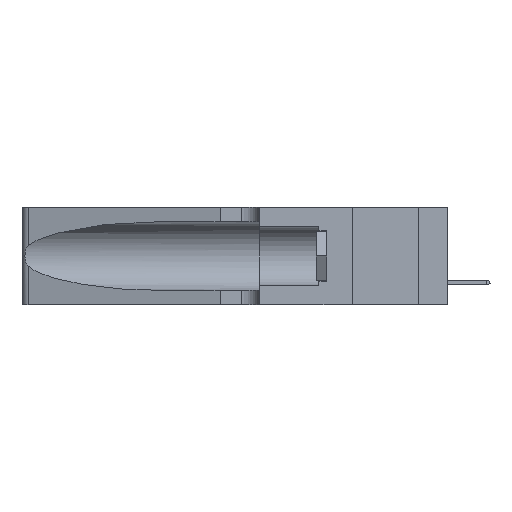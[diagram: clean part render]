
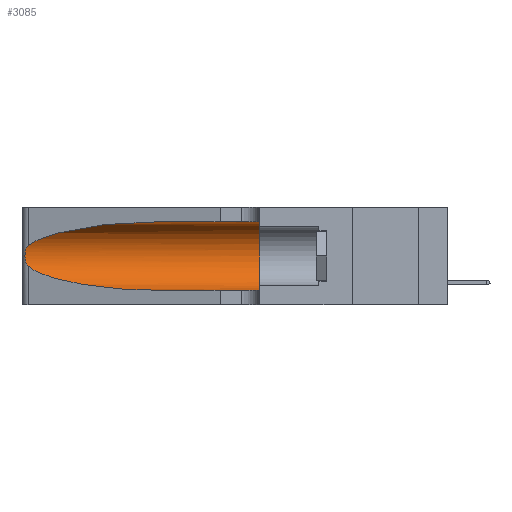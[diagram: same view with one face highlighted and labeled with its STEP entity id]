
A CAD part, left-side view. The second image highlights one B-rep face of the part: STEP entity #3085.
In plain terms, the highlighted cylindrical face has radius 3.308 mm (diameter 6.617 mm), a partial arc.
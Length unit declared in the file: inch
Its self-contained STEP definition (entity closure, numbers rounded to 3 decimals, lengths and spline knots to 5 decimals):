
#16 = CARTESIAN_POINT ( 'NONE',  ( 0.1305, 0.72297, 0.31525 ) ) ;
#90 = CARTESIAN_POINT ( 'NONE',  ( 0.25555, 1.22994, 0.2215 ) ) ;
#122 = CARTESIAN_POINT ( 'NONE',  ( 0.26018, 1.23835, 0.19895 ) ) ;
#381 = CARTESIAN_POINT ( 'NONE',  ( 0.1305, 0.72297, 0.05475 ) ) ;
#1040 = AXIS2_PLACEMENT_3D ( 'NONE', #11306, #14944, #5974 ) ;
#3085 = ADVANCED_FACE ( 'NONE', ( #10903 ), #20710, .F. ) ;
#3387 = EDGE_CURVE ( 'NONE', #22578, #42365, #36849, .T. ) ;
#4624 = DIRECTION ( 'NONE',  ( 0., -1., 0. ) ) ;
#4936 = CARTESIAN_POINT ( 'NONE',  ( 0.25789, 1.23486, 0.15765 ) ) ;
#5235 = CARTESIAN_POINT ( 'NONE',  ( 0.26075, 1.23896, 0.178 ) ) ;
#5974 = DIRECTION ( 'NONE',  ( 0., 0., -1. ) ) ;
#6119 = CARTESIAN_POINT ( 'NONE',  ( 0.25639, 1.23184, 0.21858 ) ) ;
#6278 =( BOUNDED_CURVE ( )  B_SPLINE_CURVE ( 3, ( #33936, #40013, #6441, #381 ),
 .UNSPECIFIED., .F., .F. ) 
 B_SPLINE_CURVE_WITH_KNOTS ( ( 4, 4 ),
 ( 3.44316, 4.71239 ),
 .UNSPECIFIED. ) 
 CURVE ( )  GEOMETRIC_REPRESENTATION_ITEM ( )  RATIONAL_B_SPLINE_CURVE ( ( 1., 0.87, 0.87, 1. ) ) 
 REPRESENTATION_ITEM ( '' )  );
#6441 = CARTESIAN_POINT ( 'NONE',  ( 0.18966, 0.96281, 0.05475 ) ) ;
#6988 = CARTESIAN_POINT ( 'NONE',  ( 0.18966, 0.96281, 0.31525 ) ) ;
#7153 = CARTESIAN_POINT ( 'NONE',  ( 0.2373, 1.15595, 0.28018 ) ) ;
#7646 = VERTEX_POINT ( 'NONE', #41766 ) ;
#7783 = DIRECTION ( 'NONE',  ( 0., 0., 1. ) ) ;
#8116 = CARTESIAN_POINT ( 'NONE',  ( 0.25487, 1.22718, 0.22369 ) ) ;
#9734 = EDGE_LOOP ( 'NONE', ( #28332, #10501, #30326, #34204, #14039, #30371 ) ) ;
#10501 = ORIENTED_EDGE ( 'NONE', *, *, #3387, .T. ) ;
#10881 = CARTESIAN_POINT ( 'NONE',  ( 0.1305, 0.35, 0.31525 ) ) ;
#10903 = FACE_OUTER_BOUND ( 'NONE', #9734, .T. ) ;
#10955 = CARTESIAN_POINT ( 'NONE',  ( 0.1305, 1.61858, 0.31525 ) ) ;
#11306 = CARTESIAN_POINT ( 'NONE',  ( 0.1305, 1.61858, 0.185 ) ) ;
#12125 = CIRCLE ( 'NONE', #32154, 0.13025 ) ;
#12534 = CARTESIAN_POINT ( 'NONE',  ( 0.25854, 1.2359, 0.20912 ) ) ;
#14039 = ORIENTED_EDGE ( 'NONE', *, *, #19310, .F. ) ;
#14944 = DIRECTION ( 'NONE',  ( 0., -1., 0. ) ) ;
#15349 = LINE ( 'NONE', #29283, #32809 ) ;
#15632 = CARTESIAN_POINT ( 'NONE',  ( 0.25555, 1.22993, 0.14849 ) ) ;
#17340 = CARTESIAN_POINT ( 'NONE',  ( 0.1305, 0.35, 0.185 ) ) ;
#18499 = CARTESIAN_POINT ( 'NONE',  ( 0.1305, 0.72297, 0.31525 ) ) ;
#18615 = VERTEX_POINT ( 'NONE', #10881 ) ;
#19087 = CARTESIAN_POINT ( 'NONE',  ( 0.25787, 1.23484, 0.2124 ) ) ;
#19310 = EDGE_CURVE ( 'NONE', #18615, #7646, #12125, .T. ) ;
#19911 = DIRECTION ( 'NONE',  ( 0., -1., 0. ) ) ;
#20242 = CARTESIAN_POINT ( 'NONE',  ( 0.25487, 1.22718, 0.14631 ) ) ;
#20567 = CARTESIAN_POINT ( 'NONE',  ( 0.26075, 1.23896, 0.19203 ) ) ;
#20623 = EDGE_CURVE ( 'NONE', #40345, #18615, #25537, .T. ) ;
#20710 = CYLINDRICAL_SURFACE ( 'NONE', #1040, 0.13025 ) ;
#21371 = VERTEX_POINT ( 'NONE', #37599 ) ;
#22578 = VERTEX_POINT ( 'NONE', #8116 ) ;
#23713 = EDGE_CURVE ( 'NONE', #42365, #21371, #6278, .T. ) ;
#24273 =( BOUNDED_CURVE ( )  B_SPLINE_CURVE ( 3, ( #16, #6988, #7153, #33063 ),
 .UNSPECIFIED., .F., .F. ) 
 B_SPLINE_CURVE_WITH_KNOTS ( ( 4, 4 ),
 ( 1.5708, 2.84003 ),
 .UNSPECIFIED. ) 
 CURVE ( )  GEOMETRIC_REPRESENTATION_ITEM ( )  RATIONAL_B_SPLINE_CURVE ( ( 1., 0.87, 0.87, 1. ) ) 
 REPRESENTATION_ITEM ( '' )  );
#25320 = CARTESIAN_POINT ( 'NONE',  ( 0.26017, 1.23833, 0.17102 ) ) ;
#25446 = CARTESIAN_POINT ( 'NONE',  ( 0.25487, 1.22718, 0.14631 ) ) ;
#25537 = LINE ( 'NONE', #10955, #41944 ) ;
#28332 = ORIENTED_EDGE ( 'NONE', *, *, #40671, .T. ) ;
#29283 = CARTESIAN_POINT ( 'NONE',  ( 0.1305, 1.61858, 0.05475 ) ) ;
#30326 = ORIENTED_EDGE ( 'NONE', *, *, #23713, .T. ) ;
#30371 = ORIENTED_EDGE ( 'NONE', *, *, #20623, .F. ) ;
#31306 = CARTESIAN_POINT ( 'NONE',  ( 0.25639, 1.23186, 0.15144 ) ) ;
#32154 = AXIS2_PLACEMENT_3D ( 'NONE', #17340, #40458, #7783 ) ;
#32809 = VECTOR ( 'NONE', #19911, 39.37008 ) ;
#33063 = CARTESIAN_POINT ( 'NONE',  ( 0.25487, 1.22718, 0.22369 ) ) ;
#33936 = CARTESIAN_POINT ( 'NONE',  ( 0.25487, 1.22718, 0.14631 ) ) ;
#34204 = ORIENTED_EDGE ( 'NONE', *, *, #36033, .T. ) ;
#34797 = CARTESIAN_POINT ( 'NONE',  ( 0.25487, 1.22718, 0.22369 ) ) ;
#36033 = EDGE_CURVE ( 'NONE', #21371, #7646, #15349, .T. ) ;
#36849 = B_SPLINE_CURVE_WITH_KNOTS ( 'NONE', 3,
 ( #34797, #90, #6119, #19087, #12534, #122, #20567, #5235, #25320, #41780, #4936, #31306, #15632, #25446 ),
 .UNSPECIFIED., .F., .F.,
 ( 4, 2, 2, 2, 2, 2, 4 ),
 ( 0., 0.00027, 0.00053, 0.00107, 0.0016, 0.00187, 0.00214 ),
 .UNSPECIFIED. ) ;
#37599 = CARTESIAN_POINT ( 'NONE',  ( 0.1305, 0.72297, 0.05475 ) ) ;
#40013 = CARTESIAN_POINT ( 'NONE',  ( 0.2373, 1.15595, 0.08982 ) ) ;
#40345 = VERTEX_POINT ( 'NONE', #18499 ) ;
#40458 = DIRECTION ( 'NONE',  ( 0., 1., 0. ) ) ;
#40671 = EDGE_CURVE ( 'NONE', #40345, #22578, #24273, .T. ) ;
#41766 = CARTESIAN_POINT ( 'NONE',  ( 0.1305, 0.35, 0.05475 ) ) ;
#41780 = CARTESIAN_POINT ( 'NONE',  ( 0.25856, 1.23593, 0.16098 ) ) ;
#41944 = VECTOR ( 'NONE', #4624, 39.37008 ) ;
#42365 = VERTEX_POINT ( 'NONE', #20242 ) ;
